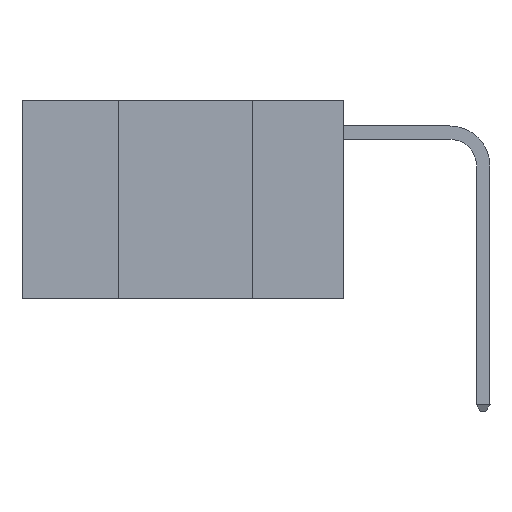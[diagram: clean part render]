
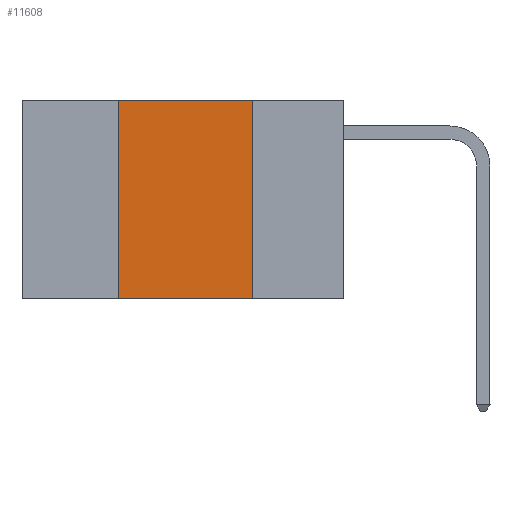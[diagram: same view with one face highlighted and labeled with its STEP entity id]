
A CAD part, left-side view. The second image highlights one B-rep face of the part: STEP entity #11608.
In plain terms, the highlighted planar face has unit normal (-1, 0, 0).
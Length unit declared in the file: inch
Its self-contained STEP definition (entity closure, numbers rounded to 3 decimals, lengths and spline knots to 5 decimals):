
#1749 = EDGE_CURVE ( 'NONE', #6457, #8934, #10393, .T. ) ;
#2348 = DIRECTION ( 'NONE',  ( 0., 0., -1. ) ) ;
#2469 = VECTOR ( 'NONE', #15978, 39.37008 ) ;
#3143 = VECTOR ( 'NONE', #23152, 39.37008 ) ;
#3681 = CARTESIAN_POINT ( 'NONE',  ( 0., 0.42, 0. ) ) ;
#3784 = DIRECTION ( 'NONE',  ( 1., 0., 0. ) ) ;
#3933 = DIRECTION ( 'NONE',  ( 0., 0., -1. ) ) ;
#4912 = CARTESIAN_POINT ( 'NONE',  ( 0., 0.6, -0.37 ) ) ;
#5245 = VERTEX_POINT ( 'NONE', #23042 ) ;
#5318 = ORIENTED_EDGE ( 'NONE', *, *, #16582, .F. ) ;
#5883 = ORIENTED_EDGE ( 'NONE', *, *, #1749, .T. ) ;
#5932 = PLANE ( 'NONE',  #22204 ) ;
#6457 = VERTEX_POINT ( 'NONE', #20811 ) ;
#7738 = LINE ( 'NONE', #10408, #14112 ) ;
#8723 = CARTESIAN_POINT ( 'NONE',  ( 0., 0.17, 0. ) ) ;
#8838 = VECTOR ( 'NONE', #2348, 39.37008 ) ;
#8934 = VERTEX_POINT ( 'NONE', #21724 ) ;
#9987 = EDGE_CURVE ( 'NONE', #6457, #16194, #14082, .T. ) ;
#10393 = LINE ( 'NONE', #4912, #3143 ) ;
#10408 = CARTESIAN_POINT ( 'NONE',  ( 0., 0.6, 0. ) ) ;
#11052 = EDGE_LOOP ( 'NONE', ( #18697, #5318, #22927, #5883 ) ) ;
#11608 = ADVANCED_FACE ( 'NONE', ( #24315 ), #5932, .F. ) ;
#12234 = CARTESIAN_POINT ( 'NONE',  ( 0., 0.42, 0. ) ) ;
#13607 = EDGE_CURVE ( 'NONE', #5245, #8934, #20900, .T. ) ;
#14082 = LINE ( 'NONE', #3681, #2469 ) ;
#14112 = VECTOR ( 'NONE', #15977, 39.37008 ) ;
#15977 = DIRECTION ( 'NONE',  ( 0., -1., 0. ) ) ;
#15978 = DIRECTION ( 'NONE',  ( 0., 0., 1. ) ) ;
#16194 = VERTEX_POINT ( 'NONE', #12234 ) ;
#16582 = EDGE_CURVE ( 'NONE', #16194, #5245, #7738, .T. ) ;
#18697 = ORIENTED_EDGE ( 'NONE', *, *, #13607, .F. ) ;
#20811 = CARTESIAN_POINT ( 'NONE',  ( 0., 0.42, -0.37 ) ) ;
#20900 = LINE ( 'NONE', #8723, #8838 ) ;
#21724 = CARTESIAN_POINT ( 'NONE',  ( 0., 0.17, -0.37 ) ) ;
#22204 = AXIS2_PLACEMENT_3D ( 'NONE', #24173, #3784, #3933 ) ;
#22927 = ORIENTED_EDGE ( 'NONE', *, *, #9987, .F. ) ;
#23042 = CARTESIAN_POINT ( 'NONE',  ( 0., 0.17, 0. ) ) ;
#23152 = DIRECTION ( 'NONE',  ( 0., -1., 0. ) ) ;
#24173 = CARTESIAN_POINT ( 'NONE',  ( 0., 0.6, 0. ) ) ;
#24315 = FACE_OUTER_BOUND ( 'NONE', #11052, .T. ) ;
